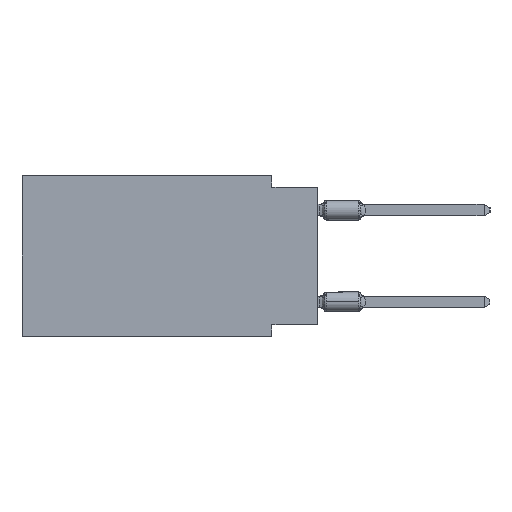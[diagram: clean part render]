
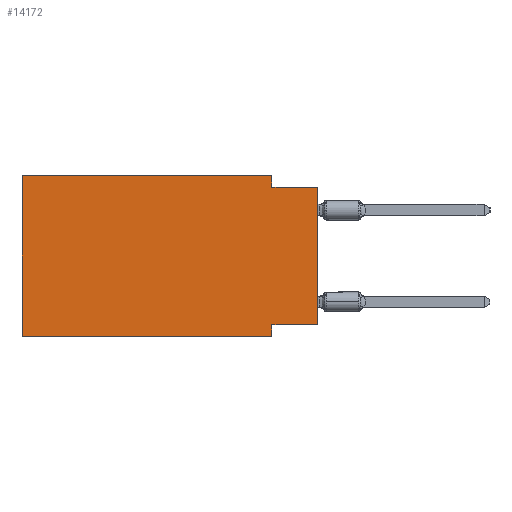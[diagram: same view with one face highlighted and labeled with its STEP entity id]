
A CAD part, left-side view. The second image highlights one B-rep face of the part: STEP entity #14172.
In plain terms, the highlighted planar face has unit normal (-1, 0, 0).
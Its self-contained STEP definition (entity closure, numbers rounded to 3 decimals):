
#276 = DIRECTION ( 'NONE',  ( 0., -1., 0. ) ) ;
#764 = CARTESIAN_POINT ( 'NONE',  ( 0., 2.54, 0. ) ) ;
#1481 = DIRECTION ( 'NONE',  ( 0., -1., 0. ) ) ;
#1492 = VECTOR ( 'NONE', #24546, 1000. ) ;
#1639 = CARTESIAN_POINT ( 'NONE',  ( 0., 0., -0.635 ) ) ;
#2458 = EDGE_CURVE ( 'NONE', #11675, #19664, #6051, .T. ) ;
#2659 = ORIENTED_EDGE ( 'NONE', *, *, #22426, .T. ) ;
#3808 = LINE ( 'NONE', #10949, #12307 ) ;
#4085 = CARTESIAN_POINT ( 'NONE',  ( 0., 0., -8.255 ) ) ;
#4588 = DIRECTION ( 'NONE',  ( 0., -1., 0. ) ) ;
#5380 = CARTESIAN_POINT ( 'NONE',  ( 0., 0., -8.255 ) ) ;
#6051 = LINE ( 'NONE', #4085, #15454 ) ;
#6141 = CARTESIAN_POINT ( 'NONE',  ( 0., 2.54, 0. ) ) ;
#6279 = EDGE_CURVE ( 'NONE', #6815, #25809, #25863, .T. ) ;
#6448 = EDGE_LOOP ( 'NONE', ( #14199, #13982, #25173, #15098, #12826, #2659, #13662, #19301 ) ) ;
#6815 = VERTEX_POINT ( 'NONE', #18005 ) ;
#6834 = VECTOR ( 'NONE', #4588, 1000. ) ;
#7059 = FACE_OUTER_BOUND ( 'NONE', #6448, .T. ) ;
#7893 = VECTOR ( 'NONE', #276, 1000. ) ;
#8833 = LINE ( 'NONE', #23768, #7893 ) ;
#8845 = DIRECTION ( 'NONE',  ( 0., 0., 1. ) ) ;
#9314 = EDGE_CURVE ( 'NONE', #19175, #6815, #19737, .T. ) ;
#9655 = EDGE_CURVE ( 'NONE', #19664, #20866, #27558, .T. ) ;
#10490 = CARTESIAN_POINT ( 'NONE',  ( 0., 16.383, 0. ) ) ;
#10949 = CARTESIAN_POINT ( 'NONE',  ( 0., 0., 0. ) ) ;
#11371 = VERTEX_POINT ( 'NONE', #17065 ) ;
#11400 = DIRECTION ( 'NONE',  ( 1., 0., 0. ) ) ;
#11675 = VERTEX_POINT ( 'NONE', #5380 ) ;
#12307 = VECTOR ( 'NONE', #8845, 1000. ) ;
#12826 = ORIENTED_EDGE ( 'NONE', *, *, #9314, .F. ) ;
#13261 = VECTOR ( 'NONE', #17085, 1000. ) ;
#13369 = CARTESIAN_POINT ( 'NONE',  ( 0., 16.383, 0. ) ) ;
#13662 = ORIENTED_EDGE ( 'NONE', *, *, #9655, .F. ) ;
#13982 = ORIENTED_EDGE ( 'NONE', *, *, #17740, .F. ) ;
#14172 = ADVANCED_FACE ( 'NONE', ( #7059 ), #21677, .F. ) ;
#14199 = ORIENTED_EDGE ( 'NONE', *, *, #26585, .T. ) ;
#14719 = DIRECTION ( 'NONE',  ( 0., 0., -1. ) ) ;
#14839 = CARTESIAN_POINT ( 'NONE',  ( 0., 16.383, -8.89 ) ) ;
#15002 = VECTOR ( 'NONE', #1481, 1000. ) ;
#15098 = ORIENTED_EDGE ( 'NONE', *, *, #6279, .F. ) ;
#15454 = VECTOR ( 'NONE', #25070, 1000. ) ;
#15484 = DIRECTION ( 'NONE',  ( 0., 0., -1. ) ) ;
#15498 = CARTESIAN_POINT ( 'NONE',  ( 0., 2.54, -8.255 ) ) ;
#16524 = LINE ( 'NONE', #1639, #15002 ) ;
#16582 = CARTESIAN_POINT ( 'NONE',  ( 0., 2.54, -0.635 ) ) ;
#17065 = CARTESIAN_POINT ( 'NONE',  ( 0., 0., -0.635 ) ) ;
#17085 = DIRECTION ( 'NONE',  ( 0., 0., -1. ) ) ;
#17740 = EDGE_CURVE ( 'NONE', #26487, #11371, #16524, .T. ) ;
#18005 = CARTESIAN_POINT ( 'NONE',  ( 0., 16.383, 0. ) ) ;
#19175 = VERTEX_POINT ( 'NONE', #14839 ) ;
#19193 = EDGE_CURVE ( 'NONE', #25809, #26487, #25433, .T. ) ;
#19301 = ORIENTED_EDGE ( 'NONE', *, *, #2458, .F. ) ;
#19664 = VERTEX_POINT ( 'NONE', #15498 ) ;
#19737 = LINE ( 'NONE', #19875, #1492 ) ;
#19875 = CARTESIAN_POINT ( 'NONE',  ( 0., 16.383, 0. ) ) ;
#20628 = CARTESIAN_POINT ( 'NONE',  ( 0., 2.54, -8.89 ) ) ;
#20866 = VERTEX_POINT ( 'NONE', #24109 ) ;
#21677 = PLANE ( 'NONE',  #24961 ) ;
#22426 = EDGE_CURVE ( 'NONE', #19175, #20866, #8833, .T. ) ;
#23768 = CARTESIAN_POINT ( 'NONE',  ( 0., 16.383, -8.89 ) ) ;
#24109 = CARTESIAN_POINT ( 'NONE',  ( 0., 2.54, -8.89 ) ) ;
#24425 = VECTOR ( 'NONE', #14719, 1000. ) ;
#24546 = DIRECTION ( 'NONE',  ( 0., 0., 1. ) ) ;
#24961 = AXIS2_PLACEMENT_3D ( 'NONE', #13369, #11400, #15484 ) ;
#25070 = DIRECTION ( 'NONE',  ( 0., 1., 0. ) ) ;
#25173 = ORIENTED_EDGE ( 'NONE', *, *, #19193, .F. ) ;
#25433 = LINE ( 'NONE', #6141, #13261 ) ;
#25809 = VERTEX_POINT ( 'NONE', #764 ) ;
#25863 = LINE ( 'NONE', #10490, #6834 ) ;
#26487 = VERTEX_POINT ( 'NONE', #16582 ) ;
#26585 = EDGE_CURVE ( 'NONE', #11675, #11371, #3808, .T. ) ;
#27558 = LINE ( 'NONE', #20628, #24425 ) ;
